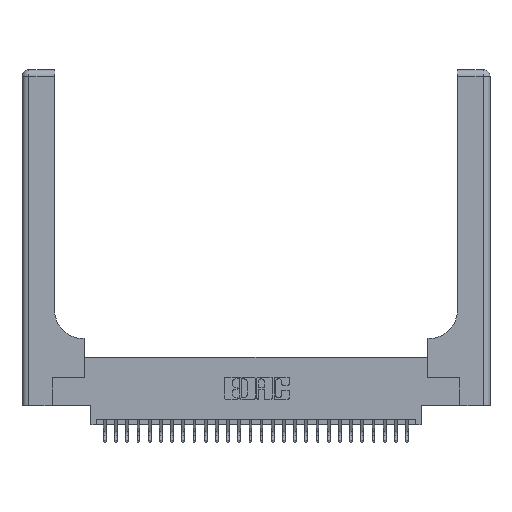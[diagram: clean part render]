
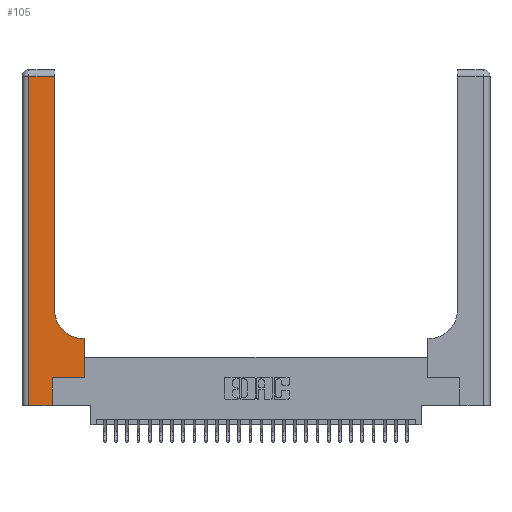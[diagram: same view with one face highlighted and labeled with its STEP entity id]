
A CAD part, top view. The second image highlights one B-rep face of the part: STEP entity #105.
In plain terms, the highlighted planar face has unit normal (0, 0, 1).
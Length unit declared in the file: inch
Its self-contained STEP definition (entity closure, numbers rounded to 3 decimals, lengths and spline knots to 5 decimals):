
#35 = ORIENTED_EDGE ( 'NONE', *, *, #9375, .T. ) ;
#105 = ADVANCED_FACE ( 'NONE', ( #22366 ), #11243, .F. ) ;
#383 = ORIENTED_EDGE ( 'NONE', *, *, #12784, .T. ) ;
#425 = VECTOR ( 'NONE', #6905, 39.37008 ) ;
#513 = CARTESIAN_POINT ( 'NONE',  ( 0.06, 3., 0.37 ) ) ;
#785 = CARTESIAN_POINT ( 'NONE',  ( 0.06, 0., 0.37 ) ) ;
#859 = DIRECTION ( 'NONE',  ( 0., 0., -1. ) ) ;
#1035 = ORIENTED_EDGE ( 'NONE', *, *, #25206, .T. ) ;
#1671 = VECTOR ( 'NONE', #1717, 39.37008 ) ;
#1717 = DIRECTION ( 'NONE',  ( 1., 0., 0. ) ) ;
#2112 = DIRECTION ( 'NONE',  ( 0., 1., 0. ) ) ;
#2150 = CARTESIAN_POINT ( 'NONE',  ( 0.2915, 2.94, 0.37 ) ) ;
#2332 = EDGE_LOOP ( 'NONE', ( #19597, #35, #4528, #14184, #24984, #383, #13777, #1035, #6002 ) ) ;
#2954 = CARTESIAN_POINT ( 'NONE',  ( 0., 2.94, 0.37 ) ) ;
#3164 = LINE ( 'NONE', #9267, #23423 ) ;
#3637 = EDGE_CURVE ( 'NONE', #24528, #18727, #3164, .T. ) ;
#4528 = ORIENTED_EDGE ( 'NONE', *, *, #24660, .T. ) ;
#4829 = DIRECTION ( 'NONE',  ( 0., -1., 0. ) ) ;
#4927 = CIRCLE ( 'NONE', #5101, 0.25 ) ;
#5101 = AXIS2_PLACEMENT_3D ( 'NONE', #25907, #859, #21546 ) ;
#5507 = VERTEX_POINT ( 'NONE', #10263 ) ;
#5929 = LINE ( 'NONE', #17416, #1671 ) ;
#6002 = ORIENTED_EDGE ( 'NONE', *, *, #15986, .T. ) ;
#6162 = LINE ( 'NONE', #2954, #20342 ) ;
#6340 = VECTOR ( 'NONE', #22595, 39.37008 ) ;
#6619 = CARTESIAN_POINT ( 'NONE',  ( 0.2915, 3., 0.37 ) ) ;
#6905 = DIRECTION ( 'NONE',  ( 0., 1., 0. ) ) ;
#7963 = VECTOR ( 'NONE', #17450, 39.37008 ) ;
#8515 = CARTESIAN_POINT ( 'NONE',  ( 0.269, 0., 0.37 ) ) ;
#9267 = CARTESIAN_POINT ( 'NONE',  ( 0.5585, 0.25, 0.37 ) ) ;
#9375 = EDGE_CURVE ( 'NONE', #26406, #5507, #6162, .T. ) ;
#9878 = VERTEX_POINT ( 'NONE', #24048 ) ;
#10263 = CARTESIAN_POINT ( 'NONE',  ( 0.06, 2.94, 0.37 ) ) ;
#11243 = PLANE ( 'NONE',  #18413 ) ;
#11443 = DIRECTION ( 'NONE',  ( 0., 0., -1. ) ) ;
#11602 = CARTESIAN_POINT ( 'NONE',  ( 0.5585, 0.6, 0.37 ) ) ;
#12784 = EDGE_CURVE ( 'NONE', #21253, #24528, #18389, .T. ) ;
#13276 = CARTESIAN_POINT ( 'NONE',  ( 0.269, 0.25, 0.37 ) ) ;
#13427 = CARTESIAN_POINT ( 'NONE',  ( 0., 3., 0.37 ) ) ;
#13567 = EDGE_CURVE ( 'NONE', #21182, #9878, #5929, .T. ) ;
#13657 = LINE ( 'NONE', #8515, #7963 ) ;
#13777 = ORIENTED_EDGE ( 'NONE', *, *, #3637, .T. ) ;
#14184 = ORIENTED_EDGE ( 'NONE', *, *, #13567, .T. ) ;
#14230 = DIRECTION ( 'NONE',  ( -1., 0., 0. ) ) ;
#14267 = LINE ( 'NONE', #513, #19595 ) ;
#15986 = EDGE_CURVE ( 'NONE', #25168, #23341, #4927, .T. ) ;
#17416 = CARTESIAN_POINT ( 'NONE',  ( 0., 0., 0.37 ) ) ;
#17450 = DIRECTION ( 'NONE',  ( 0., 1., 0. ) ) ;
#18389 = LINE ( 'NONE', #13276, #6340 ) ;
#18413 = AXIS2_PLACEMENT_3D ( 'NONE', #13427, #11443, #27317 ) ;
#18727 = VERTEX_POINT ( 'NONE', #11602 ) ;
#18831 = VECTOR ( 'NONE', #14230, 39.37008 ) ;
#18928 = LINE ( 'NONE', #6619, #425 ) ;
#19140 = EDGE_CURVE ( 'NONE', #9878, #21253, #13657, .T. ) ;
#19595 = VECTOR ( 'NONE', #4829, 39.37008 ) ;
#19597 = ORIENTED_EDGE ( 'NONE', *, *, #19850, .T. ) ;
#19850 = EDGE_CURVE ( 'NONE', #23341, #26406, #18928, .T. ) ;
#20342 = VECTOR ( 'NONE', #21229, 39.37008 ) ;
#21182 = VERTEX_POINT ( 'NONE', #785 ) ;
#21229 = DIRECTION ( 'NONE',  ( -1., 0., 0. ) ) ;
#21253 = VERTEX_POINT ( 'NONE', #23269 ) ;
#21546 = DIRECTION ( 'NONE',  ( 1., 0., 0. ) ) ;
#22366 = FACE_OUTER_BOUND ( 'NONE', #2332, .T. ) ;
#22595 = DIRECTION ( 'NONE',  ( 1., 0., 0. ) ) ;
#23067 = CARTESIAN_POINT ( 'NONE',  ( 0.2915, 0.6, 0.37 ) ) ;
#23177 = CARTESIAN_POINT ( 'NONE',  ( 0.5415, 0.6, 0.37 ) ) ;
#23269 = CARTESIAN_POINT ( 'NONE',  ( 0.269, 0.25, 0.37 ) ) ;
#23341 = VERTEX_POINT ( 'NONE', #28697 ) ;
#23423 = VECTOR ( 'NONE', #2112, 39.37008 ) ;
#24048 = CARTESIAN_POINT ( 'NONE',  ( 0.269, 0., 0.37 ) ) ;
#24528 = VERTEX_POINT ( 'NONE', #24791 ) ;
#24660 = EDGE_CURVE ( 'NONE', #5507, #21182, #14267, .T. ) ;
#24791 = CARTESIAN_POINT ( 'NONE',  ( 0.5585, 0.25, 0.37 ) ) ;
#24984 = ORIENTED_EDGE ( 'NONE', *, *, #19140, .T. ) ;
#25168 = VERTEX_POINT ( 'NONE', #23177 ) ;
#25206 = EDGE_CURVE ( 'NONE', #18727, #25168, #27077, .T. ) ;
#25907 = CARTESIAN_POINT ( 'NONE',  ( 0.5415, 0.85, 0.37 ) ) ;
#26406 = VERTEX_POINT ( 'NONE', #2150 ) ;
#27077 = LINE ( 'NONE', #23067, #18831 ) ;
#27317 = DIRECTION ( 'NONE',  ( -1., 0., 0. ) ) ;
#28697 = CARTESIAN_POINT ( 'NONE',  ( 0.2915, 0.85, 0.37 ) ) ;
